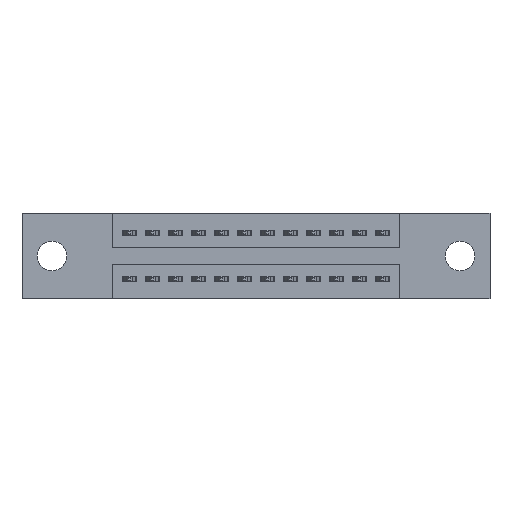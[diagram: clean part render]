
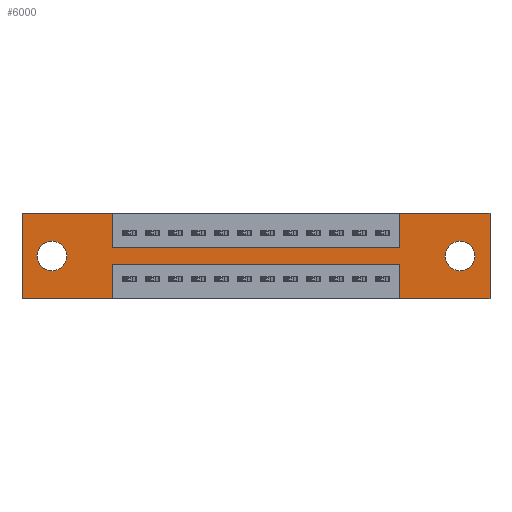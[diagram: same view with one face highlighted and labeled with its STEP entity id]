
A CAD part, front view. The second image highlights one B-rep face of the part: STEP entity #6000.
In plain terms, the highlighted planar face has unit normal (0, -1, 0).
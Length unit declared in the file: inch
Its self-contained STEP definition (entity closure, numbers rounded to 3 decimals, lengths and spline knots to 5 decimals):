
#193 = EDGE_CURVE ( 'NONE', #2728, #1703, #12639, .T. ) ;
#247 = VECTOR ( 'NONE', #7818, 39.37008 ) ;
#249 = LINE ( 'NONE', #11209, #13437 ) ;
#427 = CIRCLE ( 'NONE', #12673, 0.064 ) ;
#438 = EDGE_CURVE ( 'NONE', #3903, #5021, #6104, .T. ) ;
#546 = CARTESIAN_POINT ( 'NONE',  ( 1.6425, 0., -0.22 ) ) ;
#626 = VECTOR ( 'NONE', #969, 39.37008 ) ;
#790 = VECTOR ( 'NONE', #6654, 39.37008 ) ;
#882 = VERTEX_POINT ( 'NONE', #12471 ) ;
#963 = CARTESIAN_POINT ( 'NONE',  ( 0.13, 0., -0.121 ) ) ;
#969 = DIRECTION ( 'NONE',  ( 0., 0., -1. ) ) ;
#1213 = VECTOR ( 'NONE', #5535, 39.37008 ) ;
#1352 = EDGE_CURVE ( 'NONE', #7594, #7799, #10117, .T. ) ;
#1544 = LINE ( 'NONE', #6548, #1213 ) ;
#1703 = VERTEX_POINT ( 'NONE', #6416 ) ;
#1800 = EDGE_CURVE ( 'NONE', #12477, #2728, #1544, .T. ) ;
#1925 = EDGE_CURVE ( 'NONE', #1703, #882, #6572, .T. ) ;
#1937 = EDGE_LOOP ( 'NONE', ( #10952, #3023 ) ) ;
#2075 = ORIENTED_EDGE ( 'NONE', *, *, #1925, .F. ) ;
#2106 = CARTESIAN_POINT ( 'NONE',  ( 1.6425, 0., 0. ) ) ;
#2471 = DIRECTION ( 'NONE',  ( 0., 0., -1. ) ) ;
#2478 = VECTOR ( 'NONE', #8719, 39.37008 ) ;
#2518 = ORIENTED_EDGE ( 'NONE', *, *, #12027, .F. ) ;
#2728 = VERTEX_POINT ( 'NONE', #10094 ) ;
#2747 = CARTESIAN_POINT ( 'NONE',  ( 0., 0., -0.37 ) ) ;
#3023 = ORIENTED_EDGE ( 'NONE', *, *, #3318, .T. ) ;
#3060 = CARTESIAN_POINT ( 'NONE',  ( 1.6425, 0., -0.15 ) ) ;
#3076 = CARTESIAN_POINT ( 'NONE',  ( 0., 0., 0. ) ) ;
#3122 = ORIENTED_EDGE ( 'NONE', *, *, #438, .F. ) ;
#3139 = EDGE_CURVE ( 'NONE', #3168, #10714, #8146, .T. ) ;
#3168 = VERTEX_POINT ( 'NONE', #963 ) ;
#3288 = EDGE_CURVE ( 'NONE', #10714, #3168, #6531, .T. ) ;
#3318 = EDGE_CURVE ( 'NONE', #7309, #8784, #11412, .T. ) ;
#3357 = FACE_BOUND ( 'NONE', #1937, .T. ) ;
#3462 = DIRECTION ( 'NONE',  ( 1., 0., 0. ) ) ;
#3497 = LINE ( 'NONE', #10718, #790 ) ;
#3554 = AXIS2_PLACEMENT_3D ( 'NONE', #12750, #8631, #5367 ) ;
#3596 = EDGE_CURVE ( 'NONE', #12720, #11841, #4881, .T. ) ;
#3665 = AXIS2_PLACEMENT_3D ( 'NONE', #12376, #7108, #9197 ) ;
#3666 = ORIENTED_EDGE ( 'NONE', *, *, #1352, .F. ) ;
#3674 = ORIENTED_EDGE ( 'NONE', *, *, #3288, .T. ) ;
#3775 = ORIENTED_EDGE ( 'NONE', *, *, #9181, .F. ) ;
#3806 = EDGE_LOOP ( 'NONE', ( #12482, #12306, #10457, #2075, #9109, #11868, #8708, #3122, #3775, #3666, #13304, #2518 ) ) ;
#3805 = VECTOR ( 'NONE', #8767, 39.37008 ) ;
#3886 = CARTESIAN_POINT ( 'NONE',  ( 0.3925, 0., 0. ) ) ;
#3903 = VERTEX_POINT ( 'NONE', #7524 ) ;
#4284 = DIRECTION ( 'NONE',  ( 0., 0., -1. ) ) ;
#4881 = LINE ( 'NONE', #8984, #10223 ) ;
#5021 = VERTEX_POINT ( 'NONE', #3060 ) ;
#5029 = PLANE ( 'NONE',  #3665 ) ;
#5198 = CARTESIAN_POINT ( 'NONE',  ( 0.3925, 0., -0.37 ) ) ;
#5367 = DIRECTION ( 'NONE',  ( 0., 0., -1. ) ) ;
#5535 = DIRECTION ( 'NONE',  ( 1., 0., 0. ) ) ;
#5591 = CARTESIAN_POINT ( 'NONE',  ( 1.6425, 0., -0.37 ) ) ;
#6000 = ADVANCED_FACE ( 'NONE', ( #3357, #11825, #10660 ), #5029, .T. ) ;
#6104 = LINE ( 'NONE', #8647, #9170 ) ;
#6156 = CARTESIAN_POINT ( 'NONE',  ( 0.3925, 0., -0.22 ) ) ;
#6262 = DIRECTION ( 'NONE',  ( 1., 0., 0. ) ) ;
#6416 = CARTESIAN_POINT ( 'NONE',  ( 2.035, 0., -0.37 ) ) ;
#6517 = CARTESIAN_POINT ( 'NONE',  ( 0.13, 0., -0.185 ) ) ;
#6531 = CIRCLE ( 'NONE', #13447, 0.064 ) ;
#6548 = CARTESIAN_POINT ( 'NONE',  ( 0., 0., 0. ) ) ;
#6572 = LINE ( 'NONE', #11183, #247 ) ;
#6605 = CARTESIAN_POINT ( 'NONE',  ( 0., 0., -0.37 ) ) ;
#6654 = DIRECTION ( 'NONE',  ( 0., 0., -1. ) ) ;
#6690 = ORIENTED_EDGE ( 'NONE', *, *, #3139, .T. ) ;
#6771 = EDGE_CURVE ( 'NONE', #11841, #10353, #3497, .T. ) ;
#6888 = LINE ( 'NONE', #5591, #2478 ) ;
#7108 = DIRECTION ( 'NONE',  ( 0., -1., 0. ) ) ;
#7109 = EDGE_CURVE ( 'NONE', #5021, #12477, #7572, .T. ) ;
#7159 = EDGE_CURVE ( 'NONE', #8784, #7309, #427, .T. ) ;
#7295 = CARTESIAN_POINT ( 'NONE',  ( 1.6425, 0., 0. ) ) ;
#7309 = VERTEX_POINT ( 'NONE', #10818 ) ;
#7387 = LINE ( 'NONE', #6605, #3805 ) ;
#7524 = CARTESIAN_POINT ( 'NONE',  ( 0.3925, 0., -0.15 ) ) ;
#7572 = LINE ( 'NONE', #2106, #10469 ) ;
#7594 = VERTEX_POINT ( 'NONE', #9363 ) ;
#7799 = VERTEX_POINT ( 'NONE', #3886 ) ;
#7802 = EDGE_CURVE ( 'NONE', #10017, #7594, #249, .T. ) ;
#7818 = DIRECTION ( 'NONE',  ( -1., 0., 0. ) ) ;
#7912 = AXIS2_PLACEMENT_3D ( 'NONE', #8236, #13376, #13294 ) ;
#8146 = CIRCLE ( 'NONE', #7912, 0.064 ) ;
#8236 = CARTESIAN_POINT ( 'NONE',  ( 0.13, 0., -0.185 ) ) ;
#8631 = DIRECTION ( 'NONE',  ( 0., 1., 0. ) ) ;
#8636 = DIRECTION ( 'NONE',  ( 0., 1., 0. ) ) ;
#8647 = CARTESIAN_POINT ( 'NONE',  ( 0.3925, 0., -0.15 ) ) ;
#8708 = ORIENTED_EDGE ( 'NONE', *, *, #7109, .F. ) ;
#8719 = DIRECTION ( 'NONE',  ( 0., 0., 1. ) ) ;
#8767 = DIRECTION ( 'NONE',  ( -1., 0., 0. ) ) ;
#8784 = VERTEX_POINT ( 'NONE', #9278 ) ;
#8812 = LINE ( 'NONE', #10491, #11597 ) ;
#8984 = CARTESIAN_POINT ( 'NONE',  ( 0.3925, 0., -0.22 ) ) ;
#9109 = ORIENTED_EDGE ( 'NONE', *, *, #193, .F. ) ;
#9170 = VECTOR ( 'NONE', #3462, 39.37008 ) ;
#9181 = EDGE_CURVE ( 'NONE', #7799, #3903, #8812, .T. ) ;
#9197 = DIRECTION ( 'NONE',  ( 0., 0., -1. ) ) ;
#9278 = CARTESIAN_POINT ( 'NONE',  ( 1.905, 0., -0.121 ) ) ;
#9363 = CARTESIAN_POINT ( 'NONE',  ( 0., 0., 0. ) ) ;
#9413 = EDGE_CURVE ( 'NONE', #882, #12720, #6888, .T. ) ;
#10017 = VERTEX_POINT ( 'NONE', #2747 ) ;
#10094 = CARTESIAN_POINT ( 'NONE',  ( 2.035, 0., 0. ) ) ;
#10117 = LINE ( 'NONE', #3076, #12607 ) ;
#10223 = VECTOR ( 'NONE', #13188, 39.37008 ) ;
#10353 = VERTEX_POINT ( 'NONE', #5198 ) ;
#10457 = ORIENTED_EDGE ( 'NONE', *, *, #9413, .F. ) ;
#10469 = VECTOR ( 'NONE', #11620, 39.37008 ) ;
#10491 = CARTESIAN_POINT ( 'NONE',  ( 0.3925, 0., 0. ) ) ;
#10660 = FACE_OUTER_BOUND ( 'NONE', #3806, .T. ) ;
#10714 = VERTEX_POINT ( 'NONE', #12238 ) ;
#10718 = CARTESIAN_POINT ( 'NONE',  ( 0.3925, 0., -0.37 ) ) ;
#10768 = CARTESIAN_POINT ( 'NONE',  ( 1.905, 0., -0.185 ) ) ;
#10818 = CARTESIAN_POINT ( 'NONE',  ( 1.905, 0., -0.249 ) ) ;
#10952 = ORIENTED_EDGE ( 'NONE', *, *, #7159, .T. ) ;
#11070 = DIRECTION ( 'NONE',  ( 0., 0., 1. ) ) ;
#11183 = CARTESIAN_POINT ( 'NONE',  ( 0., 0., -0.37 ) ) ;
#11209 = CARTESIAN_POINT ( 'NONE',  ( 0., 0., 0. ) ) ;
#11412 = CIRCLE ( 'NONE', #3554, 0.064 ) ;
#11494 = CARTESIAN_POINT ( 'NONE',  ( 2.035, 0., 0. ) ) ;
#11597 = VECTOR ( 'NONE', #4284, 39.37008 ) ;
#11620 = DIRECTION ( 'NONE',  ( 0., 0., 1. ) ) ;
#11825 = FACE_BOUND ( 'NONE', #12806, .T. ) ;
#11841 = VERTEX_POINT ( 'NONE', #6156 ) ;
#11868 = ORIENTED_EDGE ( 'NONE', *, *, #1800, .F. ) ;
#12027 = EDGE_CURVE ( 'NONE', #10353, #10017, #7387, .T. ) ;
#12238 = CARTESIAN_POINT ( 'NONE',  ( 0.13, 0., -0.249 ) ) ;
#12306 = ORIENTED_EDGE ( 'NONE', *, *, #3596, .F. ) ;
#12376 = CARTESIAN_POINT ( 'NONE',  ( 0., 0., -0.37 ) ) ;
#12471 = CARTESIAN_POINT ( 'NONE',  ( 1.6425, 0., -0.37 ) ) ;
#12477 = VERTEX_POINT ( 'NONE', #7295 ) ;
#12482 = ORIENTED_EDGE ( 'NONE', *, *, #6771, .F. ) ;
#12607 = VECTOR ( 'NONE', #6262, 39.37008 ) ;
#12639 = LINE ( 'NONE', #11494, #626 ) ;
#12673 = AXIS2_PLACEMENT_3D ( 'NONE', #10768, #8636, #2471 ) ;
#12710 = DIRECTION ( 'NONE',  ( 0., 1., 0. ) ) ;
#12720 = VERTEX_POINT ( 'NONE', #546 ) ;
#12750 = CARTESIAN_POINT ( 'NONE',  ( 1.905, 0., -0.185 ) ) ;
#12793 = DIRECTION ( 'NONE',  ( 0., 0., 1. ) ) ;
#12806 = EDGE_LOOP ( 'NONE', ( #6690, #3674 ) ) ;
#13188 = DIRECTION ( 'NONE',  ( -1., 0., 0. ) ) ;
#13294 = DIRECTION ( 'NONE',  ( 0., 0., 1. ) ) ;
#13304 = ORIENTED_EDGE ( 'NONE', *, *, #7802, .F. ) ;
#13376 = DIRECTION ( 'NONE',  ( 0., 1., 0. ) ) ;
#13437 = VECTOR ( 'NONE', #11070, 39.37008 ) ;
#13447 = AXIS2_PLACEMENT_3D ( 'NONE', #6517, #12710, #12793 ) ;
